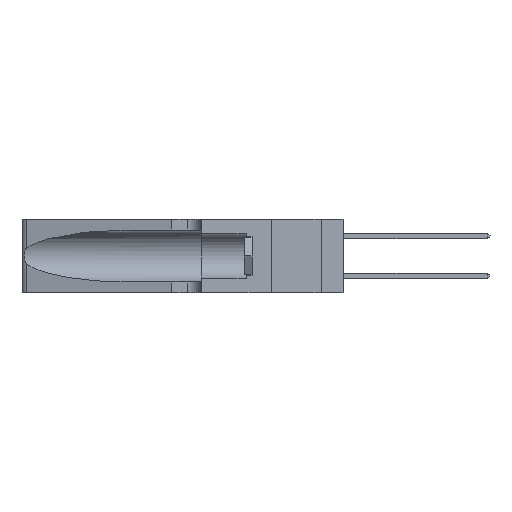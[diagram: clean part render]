
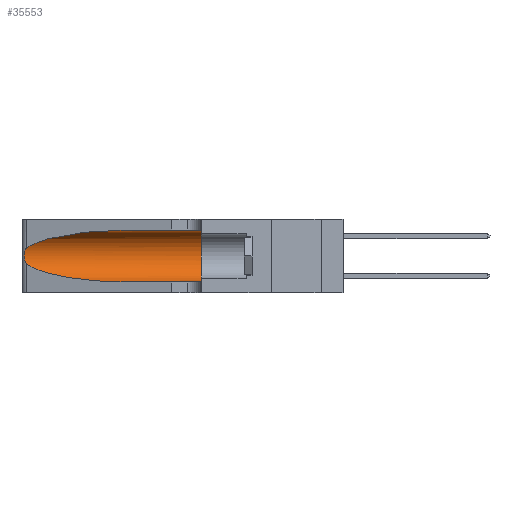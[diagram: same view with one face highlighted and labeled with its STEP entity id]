
A CAD part, left-side view. The second image highlights one B-rep face of the part: STEP entity #35553.
In plain terms, the highlighted cylindrical face has radius 3.308 mm (diameter 6.617 mm), a partial arc.
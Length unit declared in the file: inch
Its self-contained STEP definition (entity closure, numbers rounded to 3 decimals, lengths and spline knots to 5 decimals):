
#76 = CIRCLE ( 'NONE', #31970, 0.13025 ) ;
#1518 = VERTEX_POINT ( 'NONE', #45052 ) ;
#2682 = CARTESIAN_POINT ( 'NONE',  ( 0.26075, 1.23896, 0.178 ) ) ;
#2857 = CARTESIAN_POINT ( 'NONE',  ( 0.2373, 1.15595, 0.08982 ) ) ;
#6709 = VERTEX_POINT ( 'NONE', #43211 ) ;
#6908 = AXIS2_PLACEMENT_3D ( 'NONE', #9761, #46143, #46451 ) ;
#7067 = LINE ( 'NONE', #9810, #30597 ) ;
#8691 = CARTESIAN_POINT ( 'NONE',  ( 0.18966, 0.96281, 0.31525 ) ) ;
#9585 = CARTESIAN_POINT ( 'NONE',  ( 0.25555, 1.22993, 0.14849 ) ) ;
#9715 = EDGE_LOOP ( 'NONE', ( #9832, #16516, #13816, #44255, #19272, #24261 ) ) ;
#9761 = CARTESIAN_POINT ( 'NONE',  ( 0.1305, 1.61858, 0.185 ) ) ;
#9810 = CARTESIAN_POINT ( 'NONE',  ( 0.1305, 1.61858, 0.05475 ) ) ;
#9832 = ORIENTED_EDGE ( 'NONE', *, *, #37486, .T. ) ;
#13816 = ORIENTED_EDGE ( 'NONE', *, *, #45470, .T. ) ;
#14060 = CARTESIAN_POINT ( 'NONE',  ( 0.1305, 1.61858, 0.31525 ) ) ;
#16516 = ORIENTED_EDGE ( 'NONE', *, *, #33981, .T. ) ;
#17125 = CARTESIAN_POINT ( 'NONE',  ( 0.1305, 0.72297, 0.05475 ) ) ;
#17738 = CARTESIAN_POINT ( 'NONE',  ( 0.1305, 0.35, 0.185 ) ) ;
#18248 = EDGE_CURVE ( 'NONE', #18885, #40442, #7067, .T. ) ;
#18371 = CARTESIAN_POINT ( 'NONE',  ( 0.25487, 1.22718, 0.14631 ) ) ;
#18885 = VERTEX_POINT ( 'NONE', #17125 ) ;
#19272 = ORIENTED_EDGE ( 'NONE', *, *, #44528, .F. ) ;
#20602 = CARTESIAN_POINT ( 'NONE',  ( 0.26075, 1.23896, 0.19203 ) ) ;
#20747 = CARTESIAN_POINT ( 'NONE',  ( 0.26017, 1.23833, 0.17102 ) ) ;
#23044 = CARTESIAN_POINT ( 'NONE',  ( 0.1305, 0.35, 0.05475 ) ) ;
#24261 = ORIENTED_EDGE ( 'NONE', *, *, #45461, .F. ) ;
#24288 = CARTESIAN_POINT ( 'NONE',  ( 0.25856, 1.23593, 0.16098 ) ) ;
#24600 = CARTESIAN_POINT ( 'NONE',  ( 0.25854, 1.2359, 0.20912 ) ) ;
#28764 = DIRECTION ( 'NONE',  ( 0., 0., 1. ) ) ;
#28858 = CYLINDRICAL_SURFACE ( 'NONE', #6908, 0.13025 ) ;
#30597 = VECTOR ( 'NONE', #46353, 39.37008 ) ;
#30620 = CARTESIAN_POINT ( 'NONE',  ( 0.1305, 0.72297, 0.31525 ) ) ;
#31067 =( BOUNDED_CURVE ( )  B_SPLINE_CURVE ( 3, ( #30620, #8691, #39397, #31873 ),
 .UNSPECIFIED., .F., .F. ) 
 B_SPLINE_CURVE_WITH_KNOTS ( ( 4, 4 ),
 ( 1.5708, 2.84003 ),
 .UNSPECIFIED. ) 
 CURVE ( )  GEOMETRIC_REPRESENTATION_ITEM ( )  RATIONAL_B_SPLINE_CURVE ( ( 1., 0.87, 0.87, 1. ) ) 
 REPRESENTATION_ITEM ( '' )  );
#31533 = CARTESIAN_POINT ( 'NONE',  ( 0.25787, 1.23484, 0.2124 ) ) ;
#31873 = CARTESIAN_POINT ( 'NONE',  ( 0.25487, 1.22718, 0.22369 ) ) ;
#31970 = AXIS2_PLACEMENT_3D ( 'NONE', #17738, #43369, #28764 ) ;
#33120 = CARTESIAN_POINT ( 'NONE',  ( 0.25487, 1.22718, 0.22369 ) ) ;
#33510 = VERTEX_POINT ( 'NONE', #40520 ) ;
#33711 =( BOUNDED_CURVE ( )  B_SPLINE_CURVE ( 3, ( #46605, #2857, #43219, #35860 ),
 .UNSPECIFIED., .F., .F. ) 
 B_SPLINE_CURVE_WITH_KNOTS ( ( 4, 4 ),
 ( 3.44316, 4.71239 ),
 .UNSPECIFIED. ) 
 CURVE ( )  GEOMETRIC_REPRESENTATION_ITEM ( )  RATIONAL_B_SPLINE_CURVE ( ( 1., 0.87, 0.87, 1. ) ) 
 REPRESENTATION_ITEM ( '' )  );
#33981 = EDGE_CURVE ( 'NONE', #35726, #1518, #42227, .T. ) ;
#35553 = ADVANCED_FACE ( 'NONE', ( #41512 ), #28858, .F. ) ;
#35666 = CARTESIAN_POINT ( 'NONE',  ( 0.25789, 1.23486, 0.15765 ) ) ;
#35726 = VERTEX_POINT ( 'NONE', #33120 ) ;
#35860 = CARTESIAN_POINT ( 'NONE',  ( 0.1305, 0.72297, 0.05475 ) ) ;
#35931 = VECTOR ( 'NONE', #42920, 39.37008 ) ;
#37486 = EDGE_CURVE ( 'NONE', #6709, #35726, #31067, .T. ) ;
#38884 = CARTESIAN_POINT ( 'NONE',  ( 0.25639, 1.23184, 0.21858 ) ) ;
#39397 = CARTESIAN_POINT ( 'NONE',  ( 0.2373, 1.15595, 0.28018 ) ) ;
#40442 = VERTEX_POINT ( 'NONE', #23044 ) ;
#40520 = CARTESIAN_POINT ( 'NONE',  ( 0.1305, 0.35, 0.31525 ) ) ;
#41512 = FACE_OUTER_BOUND ( 'NONE', #9715, .T. ) ;
#42227 = B_SPLINE_CURVE_WITH_KNOTS ( 'NONE', 3,
 ( #42576, #46895, #38884, #31533, #24600, #46576, #20602, #2682, #20747, #24288, #35666, #46742, #9585, #18371 ),
 .UNSPECIFIED., .F., .F.,
 ( 4, 2, 2, 2, 2, 2, 4 ),
 ( 0., 0.00027, 0.00053, 0.00107, 0.0016, 0.00187, 0.00214 ),
 .UNSPECIFIED. ) ;
#42576 = CARTESIAN_POINT ( 'NONE',  ( 0.25487, 1.22718, 0.22369 ) ) ;
#42920 = DIRECTION ( 'NONE',  ( 0., -1., 0. ) ) ;
#43211 = CARTESIAN_POINT ( 'NONE',  ( 0.1305, 0.72297, 0.31525 ) ) ;
#43219 = CARTESIAN_POINT ( 'NONE',  ( 0.18966, 0.96281, 0.05475 ) ) ;
#43369 = DIRECTION ( 'NONE',  ( 0., 1., 0. ) ) ;
#44255 = ORIENTED_EDGE ( 'NONE', *, *, #18248, .T. ) ;
#44528 = EDGE_CURVE ( 'NONE', #33510, #40442, #76, .T. ) ;
#45052 = CARTESIAN_POINT ( 'NONE',  ( 0.25487, 1.22718, 0.14631 ) ) ;
#45461 = EDGE_CURVE ( 'NONE', #6709, #33510, #46840, .T. ) ;
#45470 = EDGE_CURVE ( 'NONE', #1518, #18885, #33711, .T. ) ;
#46143 = DIRECTION ( 'NONE',  ( 0., -1., 0. ) ) ;
#46353 = DIRECTION ( 'NONE',  ( 0., -1., 0. ) ) ;
#46451 = DIRECTION ( 'NONE',  ( 0., 0., -1. ) ) ;
#46576 = CARTESIAN_POINT ( 'NONE',  ( 0.26018, 1.23835, 0.19895 ) ) ;
#46605 = CARTESIAN_POINT ( 'NONE',  ( 0.25487, 1.22718, 0.14631 ) ) ;
#46742 = CARTESIAN_POINT ( 'NONE',  ( 0.25639, 1.23186, 0.15144 ) ) ;
#46840 = LINE ( 'NONE', #14060, #35931 ) ;
#46895 = CARTESIAN_POINT ( 'NONE',  ( 0.25555, 1.22994, 0.2215 ) ) ;
